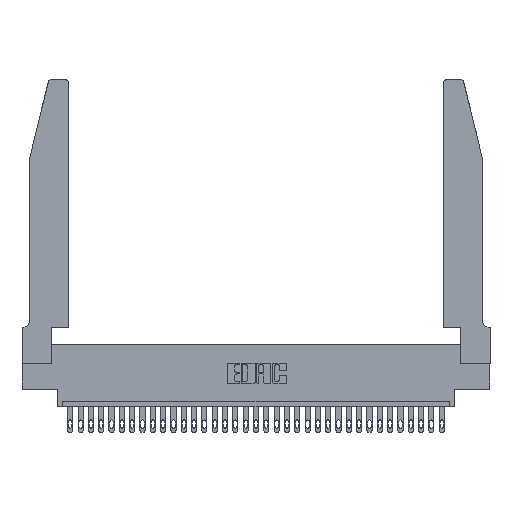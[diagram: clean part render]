
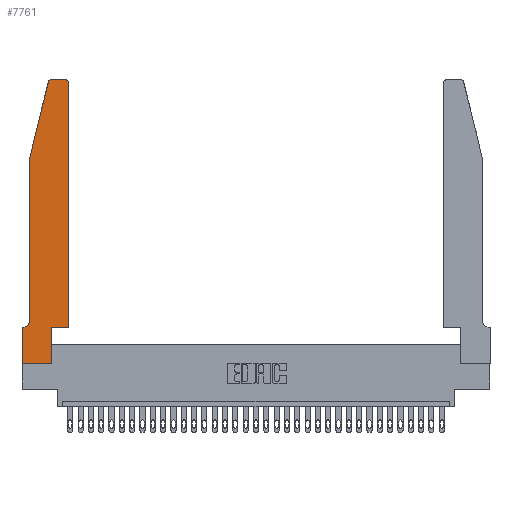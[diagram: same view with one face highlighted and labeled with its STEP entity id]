
A CAD part, top view. The second image highlights one B-rep face of the part: STEP entity #7761.
In plain terms, the highlighted planar face has unit normal (0, 0, 1).
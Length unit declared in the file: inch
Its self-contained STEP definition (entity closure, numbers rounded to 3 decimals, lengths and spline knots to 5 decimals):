
#416 = LINE ( 'NONE', #22761, #29870 ) ;
#1281 = LINE ( 'NONE', #23211, #15383 ) ;
#1692 = CARTESIAN_POINT ( 'NONE',  ( 0.4205, 2.75, 0.37 ) ) ;
#1991 = PLANE ( 'NONE',  #30367 ) ;
#2359 = CARTESIAN_POINT ( 'NONE',  ( 0., 0.35, 0.37 ) ) ;
#2832 = ORIENTED_EDGE ( 'NONE', *, *, #16052, .T. ) ;
#2904 = LINE ( 'NONE', #15764, #3699 ) ;
#3085 = ORIENTED_EDGE ( 'NONE', *, *, #8403, .T. ) ;
#3197 = CARTESIAN_POINT ( 'NONE',  ( 0.284, 2.72, 0.37 ) ) ;
#3301 = VECTOR ( 'NONE', #11482, 39.37008 ) ;
#3699 = VECTOR ( 'NONE', #8751, 39.37008 ) ;
#3752 = DIRECTION ( 'NONE',  ( 0., 1., 0. ) ) ;
#3968 = CARTESIAN_POINT ( 'NONE',  ( 0.4205, 2.72, 0.37 ) ) ;
#3994 = DIRECTION ( 'NONE',  ( 0., 0., -1. ) ) ;
#4340 = VERTEX_POINT ( 'NONE', #12895 ) ;
#4469 = VERTEX_POINT ( 'NONE', #29100 ) ;
#4481 = VERTEX_POINT ( 'NONE', #6469 ) ;
#5133 = CARTESIAN_POINT ( 'NONE',  ( 0.4505, 2.72, 0.37 ) ) ;
#5220 = ORIENTED_EDGE ( 'NONE', *, *, #28393, .T. ) ;
#5374 = VERTEX_POINT ( 'NONE', #14410 ) ;
#5672 = EDGE_CURVE ( 'NONE', #13727, #5374, #13860, .T. ) ;
#6108 = DIRECTION ( 'NONE',  ( 1., 0., 0. ) ) ;
#6317 = LINE ( 'NONE', #29648, #11097 ) ;
#6469 = CARTESIAN_POINT ( 'NONE',  ( 0.0755, 2., 0.37 ) ) ;
#6500 = LINE ( 'NONE', #10161, #8458 ) ;
#6782 = VERTEX_POINT ( 'NONE', #2359 ) ;
#7266 = FACE_OUTER_BOUND ( 'NONE', #9924, .T. ) ;
#7404 = VERTEX_POINT ( 'NONE', #5133 ) ;
#7433 = DIRECTION ( 'NONE',  ( 0., -1., 0. ) ) ;
#7761 = ADVANCED_FACE ( 'NONE', ( #7266 ), #1991, .T. ) ;
#8403 = EDGE_CURVE ( 'NONE', #20951, #6782, #2904, .T. ) ;
#8458 = VECTOR ( 'NONE', #30332, 39.37008 ) ;
#8751 = DIRECTION ( 'NONE',  ( -1., 0., 0. ) ) ;
#9370 = CIRCLE ( 'NONE', #24817, 0.03 ) ;
#9549 = ORIENTED_EDGE ( 'NONE', *, *, #19053, .T. ) ;
#9924 = EDGE_LOOP ( 'NONE', ( #23253, #9549, #31470, #19771, #30888, #3085, #2832, #29183, #5220, #10265, #23811, #29922 ) ) ;
#10145 = LINE ( 'NONE', #13739, #3301 ) ;
#10161 = CARTESIAN_POINT ( 'NONE',  ( 0.4505, 0.35, 0.37 ) ) ;
#10265 = ORIENTED_EDGE ( 'NONE', *, *, #26301, .T. ) ;
#10523 = LINE ( 'NONE', #11394, #25456 ) ;
#10729 = EDGE_CURVE ( 'NONE', #4469, #4340, #6317, .T. ) ;
#10741 = EDGE_CURVE ( 'NONE', #27114, #20951, #23608, .T. ) ;
#11097 = VECTOR ( 'NONE', #6108, 39.37008 ) ;
#11169 = VERTEX_POINT ( 'NONE', #17711 ) ;
#11185 = CARTESIAN_POINT ( 'NONE',  ( 0.0055, 0.42, 0.37 ) ) ;
#11346 = VERTEX_POINT ( 'NONE', #28787 ) ;
#11394 = CARTESIAN_POINT ( 'NONE',  ( 0.4505, 0.35, 0.37 ) ) ;
#11482 = DIRECTION ( 'NONE',  ( 0., -1., 0. ) ) ;
#12895 = CARTESIAN_POINT ( 'NONE',  ( 0.2865, 0., 0.37 ) ) ;
#13131 = DIRECTION ( 'NONE',  ( 1., 0., 0. ) ) ;
#13727 = VERTEX_POINT ( 'NONE', #1692 ) ;
#13739 = CARTESIAN_POINT ( 'NONE',  ( 0.0755, 2., 0.37 ) ) ;
#13860 = LINE ( 'NONE', #14667, #21513 ) ;
#14410 = CARTESIAN_POINT ( 'NONE',  ( 0.284, 2.75, 0.37 ) ) ;
#14667 = CARTESIAN_POINT ( 'NONE',  ( 0.2605, 2.75, 0.37 ) ) ;
#14762 = DIRECTION ( 'NONE',  ( -0.239, -0.971, 0. ) ) ;
#15383 = VECTOR ( 'NONE', #7433, 39.37008 ) ;
#15764 = CARTESIAN_POINT ( 'NONE',  ( 0.0755, 0.35, 0.37 ) ) ;
#16052 = EDGE_CURVE ( 'NONE', #6782, #4469, #1281, .T. ) ;
#17238 = DIRECTION ( 'NONE',  ( 0., 1., 0. ) ) ;
#17403 = DIRECTION ( 'NONE',  ( 1., 0., 0. ) ) ;
#17513 = DIRECTION ( 'NONE',  ( 0., 0., 1. ) ) ;
#17711 = CARTESIAN_POINT ( 'NONE',  ( 0.25487, 2.72718, 0.37 ) ) ;
#19053 = EDGE_CURVE ( 'NONE', #5374, #11169, #9370, .T. ) ;
#19128 = LINE ( 'NONE', #32708, #25900 ) ;
#19706 = EDGE_CURVE ( 'NONE', #11169, #4481, #416, .T. ) ;
#19771 = ORIENTED_EDGE ( 'NONE', *, *, #22492, .T. ) ;
#20146 = CARTESIAN_POINT ( 'NONE',  ( 0., 0.35, 0.37 ) ) ;
#20164 = VERTEX_POINT ( 'NONE', #32781 ) ;
#20951 = VERTEX_POINT ( 'NONE', #29947 ) ;
#21513 = VECTOR ( 'NONE', #31517, 39.37008 ) ;
#21810 = EDGE_CURVE ( 'NONE', #7404, #13727, #29555, .T. ) ;
#22113 = DIRECTION ( 'NONE',  ( -1., 0., 0. ) ) ;
#22469 = AXIS2_PLACEMENT_3D ( 'NONE', #3968, #17513, #17403 ) ;
#22492 = EDGE_CURVE ( 'NONE', #4481, #27114, #10145, .T. ) ;
#22514 = DIRECTION ( 'NONE',  ( 0., 0., 1. ) ) ;
#22761 = CARTESIAN_POINT ( 'NONE',  ( 0.0755, 2., 0.37 ) ) ;
#23211 = CARTESIAN_POINT ( 'NONE',  ( 0., 0., 0.37 ) ) ;
#23253 = ORIENTED_EDGE ( 'NONE', *, *, #5672, .T. ) ;
#23608 = CIRCLE ( 'NONE', #31714, 0.07 ) ;
#23806 = DIRECTION ( 'NONE',  ( 0., 0., 1. ) ) ;
#23811 = ORIENTED_EDGE ( 'NONE', *, *, #29019, .T. ) ;
#24817 = AXIS2_PLACEMENT_3D ( 'NONE', #3197, #23806, #13131 ) ;
#25227 = DIRECTION ( 'NONE',  ( 1., 0., 0. ) ) ;
#25456 = VECTOR ( 'NONE', #3752, 39.37008 ) ;
#25900 = VECTOR ( 'NONE', #17238, 39.37008 ) ;
#26301 = EDGE_CURVE ( 'NONE', #20164, #11346, #6500, .T. ) ;
#27114 = VERTEX_POINT ( 'NONE', #28896 ) ;
#28393 = EDGE_CURVE ( 'NONE', #4340, #20164, #19128, .T. ) ;
#28787 = CARTESIAN_POINT ( 'NONE',  ( 0.4505, 0.35, 0.37 ) ) ;
#28896 = CARTESIAN_POINT ( 'NONE',  ( 0.0755, 0.42, 0.37 ) ) ;
#29019 = EDGE_CURVE ( 'NONE', #11346, #7404, #10523, .T. ) ;
#29100 = CARTESIAN_POINT ( 'NONE',  ( 0., 0., 0.37 ) ) ;
#29183 = ORIENTED_EDGE ( 'NONE', *, *, #10729, .T. ) ;
#29555 = CIRCLE ( 'NONE', #22469, 0.03 ) ;
#29648 = CARTESIAN_POINT ( 'NONE',  ( 0., 0., 0.37 ) ) ;
#29870 = VECTOR ( 'NONE', #14762, 39.37008 ) ;
#29922 = ORIENTED_EDGE ( 'NONE', *, *, #21810, .T. ) ;
#29947 = CARTESIAN_POINT ( 'NONE',  ( 0.0055, 0.35, 0.37 ) ) ;
#30332 = DIRECTION ( 'NONE',  ( 1., 0., 0. ) ) ;
#30367 = AXIS2_PLACEMENT_3D ( 'NONE', #20146, #22514, #25227 ) ;
#30888 = ORIENTED_EDGE ( 'NONE', *, *, #10741, .T. ) ;
#31470 = ORIENTED_EDGE ( 'NONE', *, *, #19706, .T. ) ;
#31517 = DIRECTION ( 'NONE',  ( -1., 0., 0. ) ) ;
#31714 = AXIS2_PLACEMENT_3D ( 'NONE', #11185, #3994, #22113 ) ;
#32708 = CARTESIAN_POINT ( 'NONE',  ( 0.2865, 0.35, 0.37 ) ) ;
#32781 = CARTESIAN_POINT ( 'NONE',  ( 0.2865, 0.35, 0.37 ) ) ;
